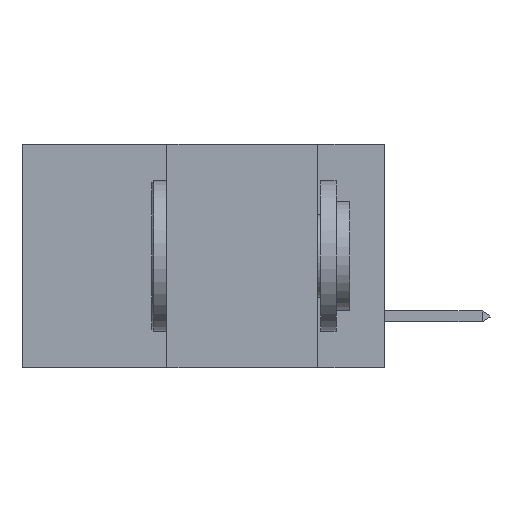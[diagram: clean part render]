
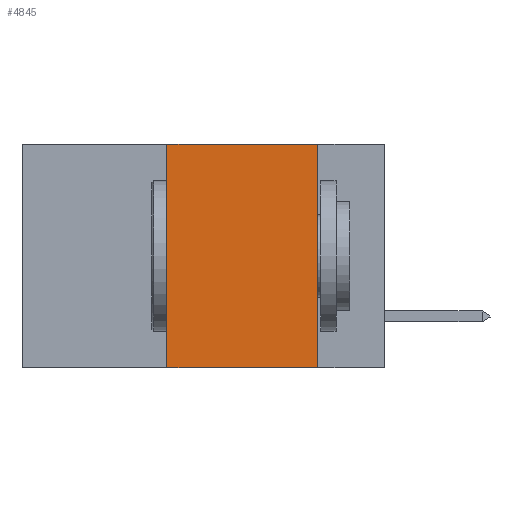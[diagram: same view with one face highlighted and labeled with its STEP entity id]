
A CAD part, left-side view. The second image highlights one B-rep face of the part: STEP entity #4845.
In plain terms, the highlighted planar face has unit normal (-1, 0, 0).
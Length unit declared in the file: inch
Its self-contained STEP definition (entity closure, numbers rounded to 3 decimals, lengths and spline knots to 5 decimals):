
#63 = DIRECTION ( 'NONE',  ( 0., -1., 0. ) ) ;
#1307 = CARTESIAN_POINT ( 'NONE',  ( 0., 0.36, -0.37 ) ) ;
#1338 = CARTESIAN_POINT ( 'NONE',  ( 0., 0.36, 0. ) ) ;
#2024 = VERTEX_POINT ( 'NONE', #13540 ) ;
#2863 = CARTESIAN_POINT ( 'NONE',  ( 0., 0.11, -0.37 ) ) ;
#4071 = LINE ( 'NONE', #12943, #13774 ) ;
#4348 = VECTOR ( 'NONE', #15682, 39.37008 ) ;
#4606 = LINE ( 'NONE', #19885, #14932 ) ;
#4636 = DIRECTION ( 'NONE',  ( 0., 0., -1. ) ) ;
#4778 = EDGE_CURVE ( 'NONE', #18845, #2024, #4606, .T. ) ;
#4845 = ADVANCED_FACE ( 'NONE', ( #18969 ), #11708, .F. ) ;
#5549 = VERTEX_POINT ( 'NONE', #1307 ) ;
#6504 = EDGE_CURVE ( 'NONE', #5549, #22170, #12319, .T. ) ;
#8589 = EDGE_LOOP ( 'NONE', ( #8939, #25039, #14754, #10890 ) ) ;
#8939 = ORIENTED_EDGE ( 'NONE', *, *, #12188, .F. ) ;
#10563 = DIRECTION ( 'NONE',  ( 0., 0., -1. ) ) ;
#10668 = DIRECTION ( 'NONE',  ( 1., 0., 0. ) ) ;
#10785 = CARTESIAN_POINT ( 'NONE',  ( 0., 0.6, 0. ) ) ;
#10890 = ORIENTED_EDGE ( 'NONE', *, *, #6504, .T. ) ;
#11433 = AXIS2_PLACEMENT_3D ( 'NONE', #10785, #10668, #10563 ) ;
#11680 = VECTOR ( 'NONE', #63, 39.37008 ) ;
#11708 = PLANE ( 'NONE',  #11433 ) ;
#12188 = EDGE_CURVE ( 'NONE', #2024, #22170, #4071, .T. ) ;
#12319 = LINE ( 'NONE', #16540, #11680 ) ;
#12943 = CARTESIAN_POINT ( 'NONE',  ( 0., 0.11, 0. ) ) ;
#13540 = CARTESIAN_POINT ( 'NONE',  ( 0., 0.11, 0. ) ) ;
#13774 = VECTOR ( 'NONE', #4636, 39.37008 ) ;
#14754 = ORIENTED_EDGE ( 'NONE', *, *, #17782, .F. ) ;
#14932 = VECTOR ( 'NONE', #18304, 39.37008 ) ;
#15305 = LINE ( 'NONE', #1338, #4348 ) ;
#15682 = DIRECTION ( 'NONE',  ( 0., 0., 1. ) ) ;
#16540 = CARTESIAN_POINT ( 'NONE',  ( 0., 0.6, -0.37 ) ) ;
#17285 = CARTESIAN_POINT ( 'NONE',  ( 0., 0.36, 0. ) ) ;
#17782 = EDGE_CURVE ( 'NONE', #5549, #18845, #15305, .T. ) ;
#18304 = DIRECTION ( 'NONE',  ( 0., -1., 0. ) ) ;
#18845 = VERTEX_POINT ( 'NONE', #17285 ) ;
#18969 = FACE_OUTER_BOUND ( 'NONE', #8589, .T. ) ;
#19885 = CARTESIAN_POINT ( 'NONE',  ( 0., 0.6, 0. ) ) ;
#22170 = VERTEX_POINT ( 'NONE', #2863 ) ;
#25039 = ORIENTED_EDGE ( 'NONE', *, *, #4778, .F. ) ;
